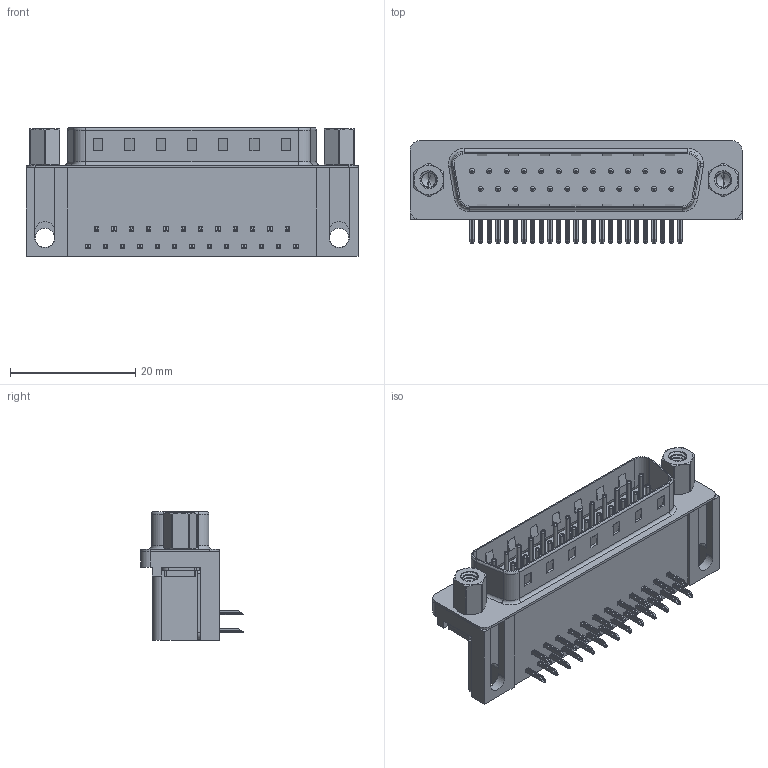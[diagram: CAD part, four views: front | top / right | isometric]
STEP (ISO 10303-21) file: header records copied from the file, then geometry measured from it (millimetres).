
FILE_DESCRIPTION (( 'STEP AP203' ), '1' );
FILE_NAME ('629-025-240-013.STEP', '2021-09-21T20:26:35', ( '' ), ( '' ), 'SwSTEP 2.0', 'SolidWorks 2020', '' );
FILE_SCHEMA (( 'CONFIG_CONTROL_DESIGN' ));
Length unit declared in the file: millimetre
Products named in the file (8): 629 Contact Bottom; 629 Thru Hole Board Mount; 629 4-40 Threaded Rivet; 629 Housing_25 Socket; 629 Shell_25 Socket; 629 4-40 Hex Standoff 5; 629 Contact Top; 629-025-240-013
Assembly tree (33 placements, depth 2):
  629-025-240-013
    629 Housing_25 Socket
    629 Shell_25 Socket
    629 Contact Bottom  x12
    629 Contact Top  x13
    629 Thru Hole Board Mount  x2
    629 4-40 Threaded Rivet  x2
    629 4-40 Hex Standoff 5  x2
Bounding box: 53.04 x 16.35 x 20.6 mm (x, y, z)
Volume: 7535.4 mm3; surface area: 8697.3 mm2
Topology: 33 solids, 33 shells, 2387 faces, 5951 edges, 3687 vertices
Faces by surface type: plane 1425, cylinder 731, torus 181, cone 32, bspline 18
Entity records: 27340 total; most frequent: CARTESIAN_POINT 8397, DIRECTION 3615, ORIENTED_EDGE 3602, EDGE_CURVE 1801, AXIS2_PLACEMENT_3D 1207, VECTOR 1201, LINE 1201, VERTEX_POINT 1158
